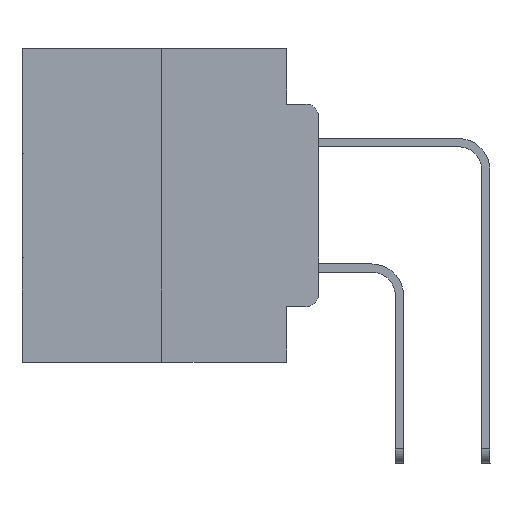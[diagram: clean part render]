
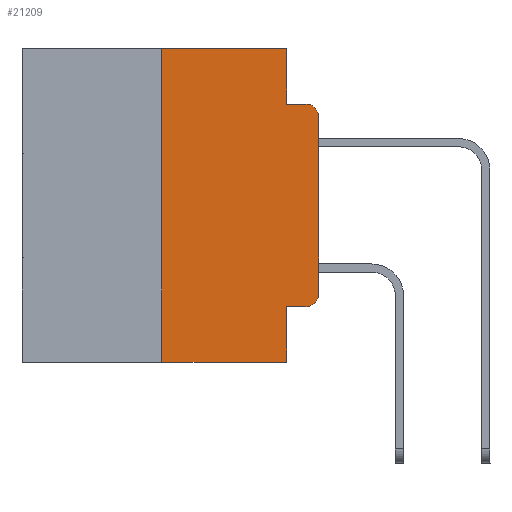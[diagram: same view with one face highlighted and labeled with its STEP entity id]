
A CAD part, left-side view. The second image highlights one B-rep face of the part: STEP entity #21209.
In plain terms, the highlighted planar face has unit normal (-1, 0, 0).
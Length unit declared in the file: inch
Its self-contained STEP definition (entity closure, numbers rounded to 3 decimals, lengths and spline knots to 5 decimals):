
#880 = EDGE_CURVE ( 'NONE', #20897, #1429, #27254, .T. ) ;
#899 = VERTEX_POINT ( 'NONE', #16915 ) ;
#1081 = DIRECTION ( 'NONE',  ( 0., 0., -1. ) ) ;
#1429 = VERTEX_POINT ( 'NONE', #16492 ) ;
#1505 = EDGE_CURVE ( 'NONE', #6638, #899, #12067, .T. ) ;
#1771 = CARTESIAN_POINT ( 'NONE',  ( 0., 0.051, 0. ) ) ;
#2191 = CARTESIAN_POINT ( 'NONE',  ( 0., 0.25, -0.5 ) ) ;
#2919 = ORIENTED_EDGE ( 'NONE', *, *, #24061, .F. ) ;
#3200 = CIRCLE ( 'NONE', #5611, 0.02 ) ;
#3988 = VECTOR ( 'NONE', #7911, 39.37008 ) ;
#4130 = EDGE_CURVE ( 'NONE', #25776, #20897, #19898, .T. ) ;
#4508 = CARTESIAN_POINT ( 'NONE',  ( 0., 0.02, -0.1085 ) ) ;
#4606 = CARTESIAN_POINT ( 'NONE',  ( 0., 0.473, 0. ) ) ;
#5142 = ORIENTED_EDGE ( 'NONE', *, *, #6276, .F. ) ;
#5611 = AXIS2_PLACEMENT_3D ( 'NONE', #28042, #14973, #1081 ) ;
#5686 = EDGE_CURVE ( 'NONE', #28340, #1429, #21493, .T. ) ;
#6161 = VECTOR ( 'NONE', #22331, 39.37008 ) ;
#6276 = EDGE_CURVE ( 'NONE', #6638, #11391, #28918, .T. ) ;
#6520 = DIRECTION ( 'NONE',  ( 0., 0., -1. ) ) ;
#6638 = VERTEX_POINT ( 'NONE', #20961 ) ;
#6871 = DIRECTION ( 'NONE',  ( 0., 0., -1. ) ) ;
#6984 = DIRECTION ( 'NONE',  ( 1., 0., 0. ) ) ;
#7351 = ORIENTED_EDGE ( 'NONE', *, *, #24236, .F. ) ;
#7490 = CARTESIAN_POINT ( 'NONE',  ( 0., 0.051, 0. ) ) ;
#7701 = ORIENTED_EDGE ( 'NONE', *, *, #880, .F. ) ;
#7798 = CARTESIAN_POINT ( 'NONE',  ( 0., 0.051, -0.5 ) ) ;
#7911 = DIRECTION ( 'NONE',  ( 0., 0., 1. ) ) ;
#9367 = VERTEX_POINT ( 'NONE', #21940 ) ;
#9631 = CARTESIAN_POINT ( 'NONE',  ( 0., 0.051, 0. ) ) ;
#10477 = VERTEX_POINT ( 'NONE', #2191 ) ;
#11391 = VERTEX_POINT ( 'NONE', #7798 ) ;
#11429 = VECTOR ( 'NONE', #24435, 39.37008 ) ;
#11795 = CARTESIAN_POINT ( 'NONE',  ( 0., 0.25, 0. ) ) ;
#11990 = ORIENTED_EDGE ( 'NONE', *, *, #21108, .T. ) ;
#12067 = LINE ( 'NONE', #14047, #23101 ) ;
#12275 = LINE ( 'NONE', #13448, #6161 ) ;
#12330 = ORIENTED_EDGE ( 'NONE', *, *, #20818, .T. ) ;
#13177 = LINE ( 'NONE', #11795, #24878 ) ;
#13448 = CARTESIAN_POINT ( 'NONE',  ( 0., 0.473, -0.5 ) ) ;
#14047 = CARTESIAN_POINT ( 'NONE',  ( 0., 0.051, -0.4115 ) ) ;
#14614 = VERTEX_POINT ( 'NONE', #29033 ) ;
#14645 = ORIENTED_EDGE ( 'NONE', *, *, #5686, .T. ) ;
#14871 = EDGE_LOOP ( 'NONE', ( #12330, #14645, #7701, #15380, #2919, #7351, #11990, #5142, #23040, #21031 ) ) ;
#14973 = DIRECTION ( 'NONE',  ( -1., 0., 0. ) ) ;
#15380 = ORIENTED_EDGE ( 'NONE', *, *, #4130, .F. ) ;
#16206 = DIRECTION ( 'NONE',  ( 0., -1., 0. ) ) ;
#16307 = CARTESIAN_POINT ( 'NONE',  ( 0., 0., -0.1085 ) ) ;
#16492 = CARTESIAN_POINT ( 'NONE',  ( 0., 0.02, -0.0885 ) ) ;
#16915 = CARTESIAN_POINT ( 'NONE',  ( 0., 0.02, -0.4115 ) ) ;
#17251 = CARTESIAN_POINT ( 'NONE',  ( 0., 0.051, -0.0885 ) ) ;
#17453 = DIRECTION ( 'NONE',  ( 0., -1., 0. ) ) ;
#17941 = CARTESIAN_POINT ( 'NONE',  ( 0., 0.473, 0. ) ) ;
#18027 = AXIS2_PLACEMENT_3D ( 'NONE', #4606, #6984, #22609 ) ;
#18111 = AXIS2_PLACEMENT_3D ( 'NONE', #4508, #20349, #6871 ) ;
#18154 = LINE ( 'NONE', #17941, #11429 ) ;
#18288 = PLANE ( 'NONE',  #18027 ) ;
#19144 = CARTESIAN_POINT ( 'NONE',  ( 0., 0., 0. ) ) ;
#19898 = LINE ( 'NONE', #7490, #24961 ) ;
#20349 = DIRECTION ( 'NONE',  ( -1., 0., 0. ) ) ;
#20818 = EDGE_CURVE ( 'NONE', #14614, #28340, #21315, .T. ) ;
#20897 = VERTEX_POINT ( 'NONE', #17251 ) ;
#20961 = CARTESIAN_POINT ( 'NONE',  ( 0., 0.051, -0.4115 ) ) ;
#21031 = ORIENTED_EDGE ( 'NONE', *, *, #22056, .T. ) ;
#21108 = EDGE_CURVE ( 'NONE', #10477, #11391, #12275, .T. ) ;
#21209 = ADVANCED_FACE ( 'NONE', ( #21283 ), #18288, .F. ) ;
#21283 = FACE_OUTER_BOUND ( 'NONE', #14871, .T. ) ;
#21315 = LINE ( 'NONE', #19144, #3988 ) ;
#21493 = CIRCLE ( 'NONE', #18111, 0.02 ) ;
#21940 = CARTESIAN_POINT ( 'NONE',  ( 0., 0.25, 0. ) ) ;
#22056 = EDGE_CURVE ( 'NONE', #899, #14614, #3200, .T. ) ;
#22331 = DIRECTION ( 'NONE',  ( 0., -1., 0. ) ) ;
#22553 = CARTESIAN_POINT ( 'NONE',  ( 0., 0.051, -0.0885 ) ) ;
#22609 = DIRECTION ( 'NONE',  ( 0., 0., -1. ) ) ;
#23040 = ORIENTED_EDGE ( 'NONE', *, *, #1505, .T. ) ;
#23043 = DIRECTION ( 'NONE',  ( 0., 0., -1. ) ) ;
#23101 = VECTOR ( 'NONE', #16206, 39.37008 ) ;
#24061 = EDGE_CURVE ( 'NONE', #9367, #25776, #18154, .T. ) ;
#24236 = EDGE_CURVE ( 'NONE', #10477, #9367, #13177, .T. ) ;
#24435 = DIRECTION ( 'NONE',  ( 0., -1., 0. ) ) ;
#24878 = VECTOR ( 'NONE', #27189, 39.37008 ) ;
#24961 = VECTOR ( 'NONE', #23043, 39.37008 ) ;
#25776 = VERTEX_POINT ( 'NONE', #9631 ) ;
#26534 = VECTOR ( 'NONE', #17453, 39.37008 ) ;
#27189 = DIRECTION ( 'NONE',  ( 0., 0., 1. ) ) ;
#27254 = LINE ( 'NONE', #22553, #26534 ) ;
#28042 = CARTESIAN_POINT ( 'NONE',  ( 0., 0.02, -0.3915 ) ) ;
#28237 = VECTOR ( 'NONE', #6520, 39.37008 ) ;
#28340 = VERTEX_POINT ( 'NONE', #16307 ) ;
#28918 = LINE ( 'NONE', #1771, #28237 ) ;
#29033 = CARTESIAN_POINT ( 'NONE',  ( 0., 0., -0.3915 ) ) ;
